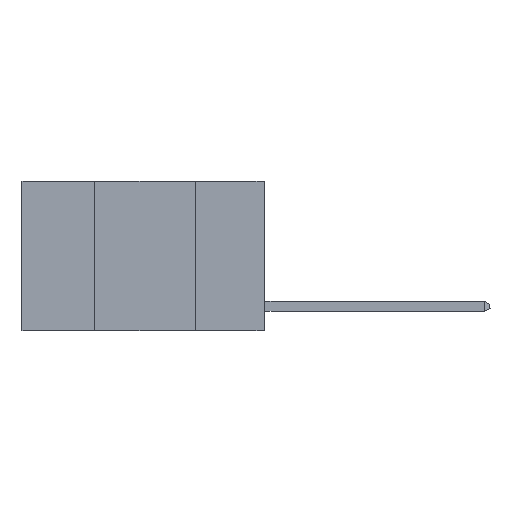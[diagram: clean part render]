
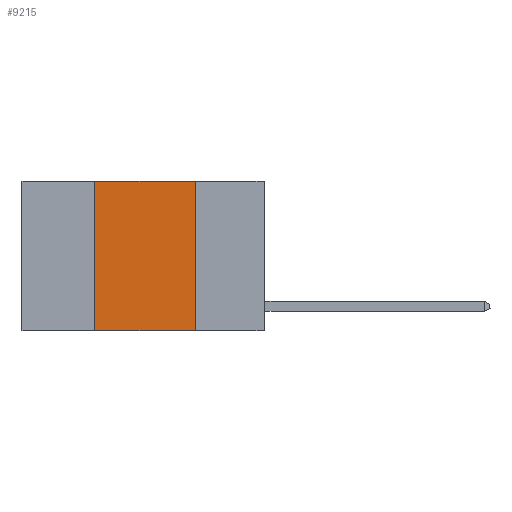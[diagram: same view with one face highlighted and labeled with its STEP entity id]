
A CAD part, left-side view. The second image highlights one B-rep face of the part: STEP entity #9215.
In plain terms, the highlighted planar face has unit normal (-1, 0, 0).
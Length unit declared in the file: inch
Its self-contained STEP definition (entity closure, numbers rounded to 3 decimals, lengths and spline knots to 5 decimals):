
#240 = VERTEX_POINT ( 'NONE', #960 ) ;
#358 = LINE ( 'NONE', #2768, #7533 ) ;
#651 = VECTOR ( 'NONE', #5640, 39.37008 ) ;
#788 = VECTOR ( 'NONE', #7601, 39.37008 ) ;
#934 = CARTESIAN_POINT ( 'NONE',  ( 0., 0.42, 0. ) ) ;
#960 = CARTESIAN_POINT ( 'NONE',  ( 0., 0.17, -0.37 ) ) ;
#965 = CARTESIAN_POINT ( 'NONE',  ( 0., 0.42, -0.37 ) ) ;
#1293 = EDGE_CURVE ( 'NONE', #11220, #240, #8972, .T. ) ;
#1945 = CARTESIAN_POINT ( 'NONE',  ( 0., 0.6, 0. ) ) ;
#1975 = CARTESIAN_POINT ( 'NONE',  ( 0., 0.6, 0. ) ) ;
#2419 = EDGE_CURVE ( 'NONE', #8777, #7852, #14463, .T. ) ;
#2768 = CARTESIAN_POINT ( 'NONE',  ( 0., 0.6, -0.37 ) ) ;
#2986 = DIRECTION ( 'NONE',  ( 0., -1., 0. ) ) ;
#3353 = DIRECTION ( 'NONE',  ( 0., 0., -1. ) ) ;
#3503 = CARTESIAN_POINT ( 'NONE',  ( 0., 0.17, 0. ) ) ;
#4436 = DIRECTION ( 'NONE',  ( 1., 0., 0. ) ) ;
#5361 = VECTOR ( 'NONE', #12096, 39.37008 ) ;
#5640 = DIRECTION ( 'NONE',  ( 0., 0., -1. ) ) ;
#5686 = ORIENTED_EDGE ( 'NONE', *, *, #1293, .F. ) ;
#7442 = CARTESIAN_POINT ( 'NONE',  ( 0., 0.42, 0. ) ) ;
#7533 = VECTOR ( 'NONE', #2986, 39.37008 ) ;
#7601 = DIRECTION ( 'NONE',  ( 0., -1., 0. ) ) ;
#7757 = ORIENTED_EDGE ( 'NONE', *, *, #14813, .F. ) ;
#7852 = VERTEX_POINT ( 'NONE', #934 ) ;
#8777 = VERTEX_POINT ( 'NONE', #965 ) ;
#8972 = LINE ( 'NONE', #14970, #651 ) ;
#9024 = FACE_OUTER_BOUND ( 'NONE', #13290, .T. ) ;
#9215 = ADVANCED_FACE ( 'NONE', ( #9024 ), #11575, .F. ) ;
#9353 = ORIENTED_EDGE ( 'NONE', *, *, #2419, .F. ) ;
#10487 = EDGE_CURVE ( 'NONE', #8777, #240, #358, .T. ) ;
#11070 = AXIS2_PLACEMENT_3D ( 'NONE', #1975, #4436, #3353 ) ;
#11220 = VERTEX_POINT ( 'NONE', #3503 ) ;
#11575 = PLANE ( 'NONE',  #11070 ) ;
#12096 = DIRECTION ( 'NONE',  ( 0., 0., 1. ) ) ;
#12541 = LINE ( 'NONE', #1945, #788 ) ;
#13290 = EDGE_LOOP ( 'NONE', ( #5686, #7757, #9353, #13705 ) ) ;
#13705 = ORIENTED_EDGE ( 'NONE', *, *, #10487, .T. ) ;
#14463 = LINE ( 'NONE', #7442, #5361 ) ;
#14813 = EDGE_CURVE ( 'NONE', #7852, #11220, #12541, .T. ) ;
#14970 = CARTESIAN_POINT ( 'NONE',  ( 0., 0.17, 0. ) ) ;
